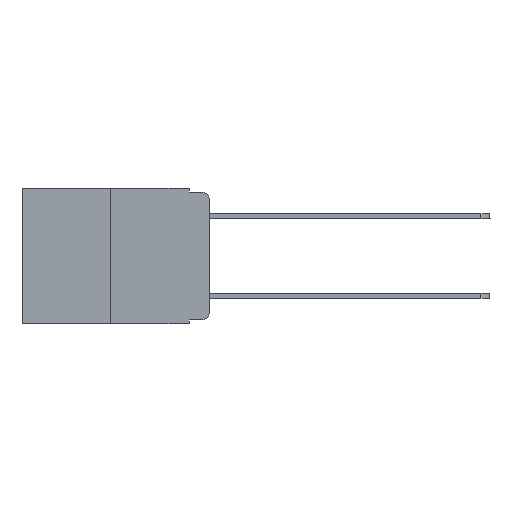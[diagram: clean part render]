
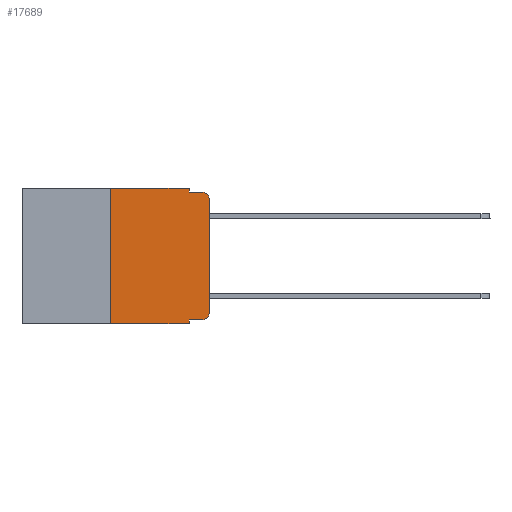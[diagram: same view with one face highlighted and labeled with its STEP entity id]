
A CAD part, left-side view. The second image highlights one B-rep face of the part: STEP entity #17689.
In plain terms, the highlighted planar face has unit normal (-1, 0, 0).
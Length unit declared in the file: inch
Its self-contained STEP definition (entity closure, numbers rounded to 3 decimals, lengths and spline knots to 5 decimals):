
#237 = VECTOR ( 'NONE', #3695, 39.37008 ) ;
#692 = DIRECTION ( 'NONE',  ( 0., 0., 1. ) ) ;
#952 = EDGE_CURVE ( 'NONE', #6549, #6847, #11401, .T. ) ;
#1264 = VERTEX_POINT ( 'NONE', #9147 ) ;
#1397 = VERTEX_POINT ( 'NONE', #9263 ) ;
#1497 = CIRCLE ( 'NONE', #9001, 0.02 ) ;
#2611 = CARTESIAN_POINT ( 'NONE',  ( 0., 0.473, 0. ) ) ;
#2795 = FACE_OUTER_BOUND ( 'NONE', #22612, .T. ) ;
#2861 = VERTEX_POINT ( 'NONE', #15478 ) ;
#3127 = ORIENTED_EDGE ( 'NONE', *, *, #8293, .F. ) ;
#3223 = DIRECTION ( 'NONE',  ( 0., 0., -1. ) ) ;
#3628 = CARTESIAN_POINT ( 'NONE',  ( 0., 0.25, 0. ) ) ;
#3695 = DIRECTION ( 'NONE',  ( 0., 0., 1. ) ) ;
#4797 = LINE ( 'NONE', #15142, #18410 ) ;
#4851 = DIRECTION ( 'NONE',  ( 0., 0., -1. ) ) ;
#4932 = CARTESIAN_POINT ( 'NONE',  ( 0., 0.25, -0.343 ) ) ;
#5263 = DIRECTION ( 'NONE',  ( 0., -1., 0. ) ) ;
#5384 = LINE ( 'NONE', #8792, #16938 ) ;
#5655 = ORIENTED_EDGE ( 'NONE', *, *, #16011, .T. ) ;
#6016 = AXIS2_PLACEMENT_3D ( 'NONE', #6930, #14077, #19494 ) ;
#6067 = ORIENTED_EDGE ( 'NONE', *, *, #22388, .T. ) ;
#6497 = VERTEX_POINT ( 'NONE', #14424 ) ;
#6516 = CARTESIAN_POINT ( 'NONE',  ( 0., 0.051, -0.333 ) ) ;
#6549 = VERTEX_POINT ( 'NONE', #3628 ) ;
#6690 = CARTESIAN_POINT ( 'NONE',  ( 0., 0., -0.03 ) ) ;
#6847 = VERTEX_POINT ( 'NONE', #20761 ) ;
#6930 = CARTESIAN_POINT ( 'NONE',  ( 0., 0.02, -0.313 ) ) ;
#7116 = CARTESIAN_POINT ( 'NONE',  ( 0., 0.051, 0. ) ) ;
#7132 = VECTOR ( 'NONE', #20827, 39.37008 ) ;
#7151 = CARTESIAN_POINT ( 'NONE',  ( 0., 0.051, -0.333 ) ) ;
#7396 = VECTOR ( 'NONE', #5263, 39.37008 ) ;
#7971 = DIRECTION ( 'NONE',  ( 1., 0., 0. ) ) ;
#8024 = EDGE_CURVE ( 'NONE', #2861, #22595, #4797, .T. ) ;
#8086 = CARTESIAN_POINT ( 'NONE',  ( 0., 0.473, 0. ) ) ;
#8103 = DIRECTION ( 'NONE',  ( 0., -1., 0. ) ) ;
#8173 = VERTEX_POINT ( 'NONE', #6690 ) ;
#8293 = EDGE_CURVE ( 'NONE', #6847, #2861, #5384, .T. ) ;
#8381 = CARTESIAN_POINT ( 'NONE',  ( 0., 0.473, -0.343 ) ) ;
#8792 = CARTESIAN_POINT ( 'NONE',  ( 0., 0.051, 0. ) ) ;
#9001 = AXIS2_PLACEMENT_3D ( 'NONE', #12107, #20949, #4851 ) ;
#9025 = ORIENTED_EDGE ( 'NONE', *, *, #12440, .F. ) ;
#9147 = CARTESIAN_POINT ( 'NONE',  ( 0., 0.051, -0.343 ) ) ;
#9263 = CARTESIAN_POINT ( 'NONE',  ( 0., 0.02, -0.333 ) ) ;
#9811 = EDGE_CURVE ( 'NONE', #6497, #8173, #11359, .T. ) ;
#10701 = ORIENTED_EDGE ( 'NONE', *, *, #13049, .T. ) ;
#10988 = ORIENTED_EDGE ( 'NONE', *, *, #9811, .T. ) ;
#11359 = LINE ( 'NONE', #18524, #17337 ) ;
#11401 = LINE ( 'NONE', #2611, #14105 ) ;
#12107 = CARTESIAN_POINT ( 'NONE',  ( 0., 0.02, -0.03 ) ) ;
#12228 = LINE ( 'NONE', #8381, #7132 ) ;
#12379 = LINE ( 'NONE', #7116, #18319 ) ;
#12440 = EDGE_CURVE ( 'NONE', #21013, #6549, #18696, .T. ) ;
#13049 = EDGE_CURVE ( 'NONE', #15111, #1397, #19592, .T. ) ;
#14077 = DIRECTION ( 'NONE',  ( -1., 0., 0. ) ) ;
#14105 = VECTOR ( 'NONE', #14814, 39.37008 ) ;
#14112 = ORIENTED_EDGE ( 'NONE', *, *, #19449, .F. ) ;
#14424 = CARTESIAN_POINT ( 'NONE',  ( 0., 0., -0.313 ) ) ;
#14814 = DIRECTION ( 'NONE',  ( 0., -1., 0. ) ) ;
#15111 = VERTEX_POINT ( 'NONE', #6516 ) ;
#15142 = CARTESIAN_POINT ( 'NONE',  ( 0., 0.051, -0.01 ) ) ;
#15237 = DIRECTION ( 'NONE',  ( 0., 0., -1. ) ) ;
#15478 = CARTESIAN_POINT ( 'NONE',  ( 0., 0.051, -0.01 ) ) ;
#16011 = EDGE_CURVE ( 'NONE', #1397, #6497, #22125, .T. ) ;
#16578 = ORIENTED_EDGE ( 'NONE', *, *, #8024, .F. ) ;
#16938 = VECTOR ( 'NONE', #17464, 39.37008 ) ;
#17337 = VECTOR ( 'NONE', #692, 39.37008 ) ;
#17464 = DIRECTION ( 'NONE',  ( 0., 0., -1. ) ) ;
#17689 = ADVANCED_FACE ( 'NONE', ( #2795 ), #20663, .F. ) ;
#18319 = VECTOR ( 'NONE', #3223, 39.37008 ) ;
#18410 = VECTOR ( 'NONE', #8103, 39.37008 ) ;
#18524 = CARTESIAN_POINT ( 'NONE',  ( 0., 0., 0. ) ) ;
#18696 = LINE ( 'NONE', #20581, #237 ) ;
#18787 = CARTESIAN_POINT ( 'NONE',  ( 0., 0.02, -0.01 ) ) ;
#19449 = EDGE_CURVE ( 'NONE', #15111, #1264, #12379, .T. ) ;
#19494 = DIRECTION ( 'NONE',  ( 0., 0., -1. ) ) ;
#19592 = LINE ( 'NONE', #7151, #7396 ) ;
#20581 = CARTESIAN_POINT ( 'NONE',  ( 0., 0.25, 0. ) ) ;
#20663 = PLANE ( 'NONE',  #22006 ) ;
#20761 = CARTESIAN_POINT ( 'NONE',  ( 0., 0.051, 0. ) ) ;
#20827 = DIRECTION ( 'NONE',  ( 0., -1., 0. ) ) ;
#20949 = DIRECTION ( 'NONE',  ( -1., 0., 0. ) ) ;
#21013 = VERTEX_POINT ( 'NONE', #4932 ) ;
#22006 = AXIS2_PLACEMENT_3D ( 'NONE', #8086, #7971, #15237 ) ;
#22125 = CIRCLE ( 'NONE', #6016, 0.02 ) ;
#22315 = EDGE_CURVE ( 'NONE', #21013, #1264, #12228, .T. ) ;
#22388 = EDGE_CURVE ( 'NONE', #8173, #22595, #1497, .T. ) ;
#22595 = VERTEX_POINT ( 'NONE', #18787 ) ;
#22604 = ORIENTED_EDGE ( 'NONE', *, *, #22315, .T. ) ;
#22612 = EDGE_LOOP ( 'NONE', ( #10988, #6067, #16578, #3127, #22767, #9025, #22604, #14112, #10701, #5655 ) ) ;
#22767 = ORIENTED_EDGE ( 'NONE', *, *, #952, .F. ) ;
